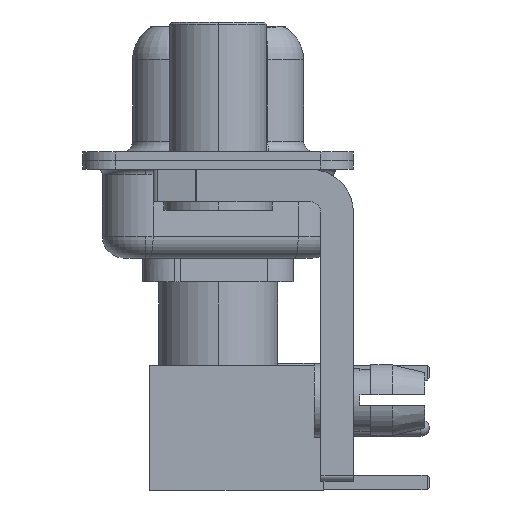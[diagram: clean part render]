
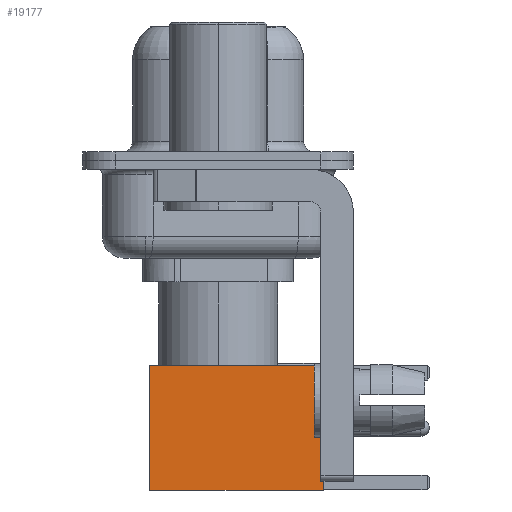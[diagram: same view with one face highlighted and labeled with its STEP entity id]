
A CAD part, left-side view. The second image highlights one B-rep face of the part: STEP entity #19177.
In plain terms, the highlighted face is planar.
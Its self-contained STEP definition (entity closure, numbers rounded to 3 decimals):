
#478 = LINE ( 'NONE', #2635, #23038 ) ;
#750 = VERTEX_POINT ( 'NONE', #6246 ) ;
#769 = VERTEX_POINT ( 'NONE', #27246 ) ;
#2635 = CARTESIAN_POINT ( 'NONE',  ( -2.875, 2.875, 0. ) ) ;
#3880 = FACE_OUTER_BOUND ( 'NONE', #12047, .T. ) ;
#5670 = ORIENTED_EDGE ( 'NONE', *, *, #22976, .F. ) ;
#5858 = VECTOR ( 'NONE', #11394, 1000. ) ;
#6246 = CARTESIAN_POINT ( 'NONE',  ( 2.875, 2.875, 8. ) ) ;
#6426 = VECTOR ( 'NONE', #21111, 1000. ) ;
#7794 = EDGE_CURVE ( 'NONE', #10652, #29250, #9575, .T. ) ;
#8465 = DIRECTION ( 'NONE',  ( 0., 1., 0. ) ) ;
#8822 = EDGE_CURVE ( 'NONE', #769, #29250, #478, .T. ) ;
#9575 = LINE ( 'NONE', #20847, #5858 ) ;
#9677 = LINE ( 'NONE', #11817, #28204 ) ;
#10652 = VERTEX_POINT ( 'NONE', #19912 ) ;
#10894 = CARTESIAN_POINT ( 'NONE',  ( 2.875, 2.875, 0. ) ) ;
#11394 = DIRECTION ( 'NONE',  ( -1., 0., 0. ) ) ;
#11817 = CARTESIAN_POINT ( 'NONE',  ( 2.875, 2.875, 0. ) ) ;
#12047 = EDGE_LOOP ( 'NONE', ( #14696, #22086, #23072, #5670 ) ) ;
#13974 = LINE ( 'NONE', #16401, #6426 ) ;
#14696 = ORIENTED_EDGE ( 'NONE', *, *, #19429, .T. ) ;
#16287 = CARTESIAN_POINT ( 'NONE',  ( -2.875, 2.875, 0. ) ) ;
#16401 = CARTESIAN_POINT ( 'NONE',  ( 0., 2.875, 8. ) ) ;
#17602 = DIRECTION ( 'NONE',  ( 0., 0., 1. ) ) ;
#19177 = ADVANCED_FACE ( 'NONE', ( #3880 ), #26623, .T. ) ;
#19429 = EDGE_CURVE ( 'NONE', #750, #10652, #9677, .T. ) ;
#19912 = CARTESIAN_POINT ( 'NONE',  ( 2.875, 2.875, 0. ) ) ;
#20847 = CARTESIAN_POINT ( 'NONE',  ( 0., 2.875, 0. ) ) ;
#21111 = DIRECTION ( 'NONE',  ( -1., 0., 0. ) ) ;
#22086 = ORIENTED_EDGE ( 'NONE', *, *, #7794, .T. ) ;
#22106 = DIRECTION ( 'NONE',  ( 0., 0., -1. ) ) ;
#22976 = EDGE_CURVE ( 'NONE', #750, #769, #13974, .T. ) ;
#23038 = VECTOR ( 'NONE', #24518, 1000. ) ;
#23072 = ORIENTED_EDGE ( 'NONE', *, *, #8822, .F. ) ;
#24518 = DIRECTION ( 'NONE',  ( 0., 0., -1. ) ) ;
#25292 = AXIS2_PLACEMENT_3D ( 'NONE', #10894, #8465, #17602 ) ;
#26623 = PLANE ( 'NONE',  #25292 ) ;
#27246 = CARTESIAN_POINT ( 'NONE',  ( -2.875, 2.875, 8. ) ) ;
#28204 = VECTOR ( 'NONE', #22106, 1000. ) ;
#29250 = VERTEX_POINT ( 'NONE', #16287 ) ;
